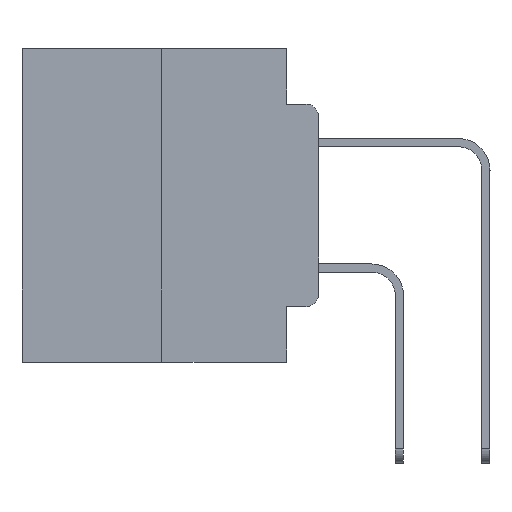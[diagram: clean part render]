
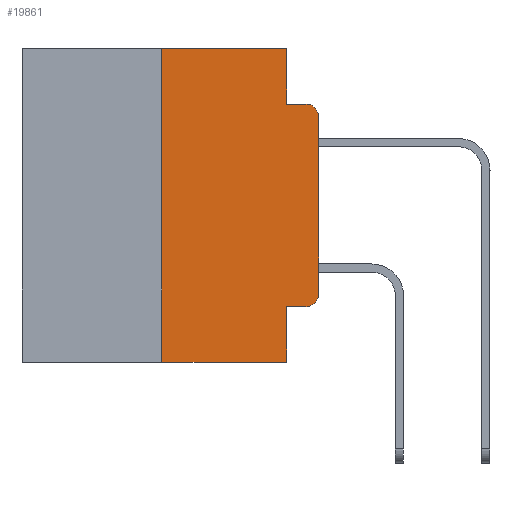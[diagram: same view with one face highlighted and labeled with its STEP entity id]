
A CAD part, left-side view. The second image highlights one B-rep face of the part: STEP entity #19861.
In plain terms, the highlighted planar face has unit normal (-1, 0, 0).
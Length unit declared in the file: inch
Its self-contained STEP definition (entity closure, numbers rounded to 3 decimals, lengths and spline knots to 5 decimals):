
#146 = VECTOR ( 'NONE', #17303, 39.37008 ) ;
#269 = ORIENTED_EDGE ( 'NONE', *, *, #26025, .T. ) ;
#361 = VERTEX_POINT ( 'NONE', #14248 ) ;
#630 = CARTESIAN_POINT ( 'NONE',  ( 0., 0.051, 0. ) ) ;
#995 = PLANE ( 'NONE',  #27758 ) ;
#1459 = CARTESIAN_POINT ( 'NONE',  ( 0., 0., 0. ) ) ;
#1549 = EDGE_CURVE ( 'NONE', #23819, #7357, #15809, .T. ) ;
#2237 = LINE ( 'NONE', #16978, #4958 ) ;
#2954 = EDGE_CURVE ( 'NONE', #18176, #9574, #23209, .T. ) ;
#3447 = CARTESIAN_POINT ( 'NONE',  ( 0., 0.473, 0. ) ) ;
#3490 = EDGE_CURVE ( 'NONE', #9643, #18176, #26949, .T. ) ;
#3621 = CARTESIAN_POINT ( 'NONE',  ( 0., 0.473, -0.5 ) ) ;
#3810 = LINE ( 'NONE', #11593, #23484 ) ;
#4132 = CARTESIAN_POINT ( 'NONE',  ( 0., 0.051, -0.5 ) ) ;
#4958 = VECTOR ( 'NONE', #10254, 39.37008 ) ;
#5354 = CARTESIAN_POINT ( 'NONE',  ( 0., 0.02, -0.0885 ) ) ;
#5599 = EDGE_CURVE ( 'NONE', #8494, #11794, #7014, .T. ) ;
#5643 = DIRECTION ( 'NONE',  ( -1., 0., 0. ) ) ;
#5781 = ORIENTED_EDGE ( 'NONE', *, *, #26069, .T. ) ;
#6562 = CARTESIAN_POINT ( 'NONE',  ( 0., 0., -0.3915 ) ) ;
#7014 = LINE ( 'NONE', #630, #26037 ) ;
#7357 = VERTEX_POINT ( 'NONE', #12744 ) ;
#7464 = ORIENTED_EDGE ( 'NONE', *, *, #3490, .F. ) ;
#7670 = VECTOR ( 'NONE', #15038, 39.37008 ) ;
#7784 = EDGE_CURVE ( 'NONE', #15511, #11794, #27935, .T. ) ;
#8494 = VERTEX_POINT ( 'NONE', #20695 ) ;
#9574 = VERTEX_POINT ( 'NONE', #5354 ) ;
#9643 = VERTEX_POINT ( 'NONE', #27072 ) ;
#9977 = ORIENTED_EDGE ( 'NONE', *, *, #17614, .T. ) ;
#10254 = DIRECTION ( 'NONE',  ( 0., -1., 0. ) ) ;
#10462 = CARTESIAN_POINT ( 'NONE',  ( 0., 0.25, -0.5 ) ) ;
#10542 = CARTESIAN_POINT ( 'NONE',  ( 0., 0.051, 0. ) ) ;
#10563 = VECTOR ( 'NONE', #16093, 39.37008 ) ;
#11404 = DIRECTION ( 'NONE',  ( 0., 0., 1. ) ) ;
#11593 = CARTESIAN_POINT ( 'NONE',  ( 0., 0.25, 0. ) ) ;
#11794 = VERTEX_POINT ( 'NONE', #4132 ) ;
#12443 = DIRECTION ( 'NONE',  ( 0., -1., 0. ) ) ;
#12705 = VERTEX_POINT ( 'NONE', #18085 ) ;
#12744 = CARTESIAN_POINT ( 'NONE',  ( 0., 0., -0.1085 ) ) ;
#12969 = EDGE_CURVE ( 'NONE', #361, #9643, #2237, .T. ) ;
#14050 = AXIS2_PLACEMENT_3D ( 'NONE', #14463, #5643, #23159 ) ;
#14248 = CARTESIAN_POINT ( 'NONE',  ( 0., 0.25, 0. ) ) ;
#14463 = CARTESIAN_POINT ( 'NONE',  ( 0., 0.02, -0.3915 ) ) ;
#15038 = DIRECTION ( 'NONE',  ( 0., 0., 1. ) ) ;
#15223 = CARTESIAN_POINT ( 'NONE',  ( 0., 0.051, -0.0885 ) ) ;
#15266 = CIRCLE ( 'NONE', #18657, 0.02 ) ;
#15511 = VERTEX_POINT ( 'NONE', #10462 ) ;
#15809 = LINE ( 'NONE', #1459, #7670 ) ;
#15832 = EDGE_CURVE ( 'NONE', #15511, #361, #3810, .T. ) ;
#16093 = DIRECTION ( 'NONE',  ( 0., -1., 0. ) ) ;
#16622 = DIRECTION ( 'NONE',  ( 0., 0., -1. ) ) ;
#16978 = CARTESIAN_POINT ( 'NONE',  ( 0., 0.473, 0. ) ) ;
#17001 = LINE ( 'NONE', #26899, #10563 ) ;
#17303 = DIRECTION ( 'NONE',  ( 0., -1., 0. ) ) ;
#17304 = DIRECTION ( 'NONE',  ( -1., 0., 0. ) ) ;
#17614 = EDGE_CURVE ( 'NONE', #7357, #9574, #15266, .T. ) ;
#18085 = CARTESIAN_POINT ( 'NONE',  ( 0., 0.02, -0.4115 ) ) ;
#18176 = VERTEX_POINT ( 'NONE', #23609 ) ;
#18657 = AXIS2_PLACEMENT_3D ( 'NONE', #21935, #17304, #19868 ) ;
#18663 = DIRECTION ( 'NONE',  ( 1., 0., 0. ) ) ;
#18799 = ORIENTED_EDGE ( 'NONE', *, *, #12969, .F. ) ;
#19820 = VECTOR ( 'NONE', #16622, 39.37008 ) ;
#19861 = ADVANCED_FACE ( 'NONE', ( #23160 ), #995, .F. ) ;
#19868 = DIRECTION ( 'NONE',  ( 0., 0., -1. ) ) ;
#20695 = CARTESIAN_POINT ( 'NONE',  ( 0., 0.051, -0.4115 ) ) ;
#21118 = ORIENTED_EDGE ( 'NONE', *, *, #5599, .F. ) ;
#21935 = CARTESIAN_POINT ( 'NONE',  ( 0., 0.02, -0.1085 ) ) ;
#22234 = ORIENTED_EDGE ( 'NONE', *, *, #2954, .F. ) ;
#22338 = DIRECTION ( 'NONE',  ( 0., 0., -1. ) ) ;
#22521 = ORIENTED_EDGE ( 'NONE', *, *, #15832, .F. ) ;
#22752 = CIRCLE ( 'NONE', #14050, 0.02 ) ;
#23159 = DIRECTION ( 'NONE',  ( 0., 0., -1. ) ) ;
#23160 = FACE_OUTER_BOUND ( 'NONE', #24434, .T. ) ;
#23209 = LINE ( 'NONE', #15223, #146 ) ;
#23484 = VECTOR ( 'NONE', #11404, 39.37008 ) ;
#23609 = CARTESIAN_POINT ( 'NONE',  ( 0., 0.051, -0.0885 ) ) ;
#23819 = VERTEX_POINT ( 'NONE', #6562 ) ;
#24434 = EDGE_LOOP ( 'NONE', ( #26295, #9977, #22234, #7464, #18799, #22521, #27981, #21118, #269, #5781 ) ) ;
#26025 = EDGE_CURVE ( 'NONE', #8494, #12705, #17001, .T. ) ;
#26037 = VECTOR ( 'NONE', #22338, 39.37008 ) ;
#26069 = EDGE_CURVE ( 'NONE', #12705, #23819, #22752, .T. ) ;
#26295 = ORIENTED_EDGE ( 'NONE', *, *, #1549, .T. ) ;
#26605 = VECTOR ( 'NONE', #12443, 39.37008 ) ;
#26899 = CARTESIAN_POINT ( 'NONE',  ( 0., 0.051, -0.4115 ) ) ;
#26949 = LINE ( 'NONE', #10542, #19820 ) ;
#26995 = DIRECTION ( 'NONE',  ( 0., 0., -1. ) ) ;
#27072 = CARTESIAN_POINT ( 'NONE',  ( 0., 0.051, 0. ) ) ;
#27758 = AXIS2_PLACEMENT_3D ( 'NONE', #3447, #18663, #26995 ) ;
#27935 = LINE ( 'NONE', #3621, #26605 ) ;
#27981 = ORIENTED_EDGE ( 'NONE', *, *, #7784, .T. ) ;
